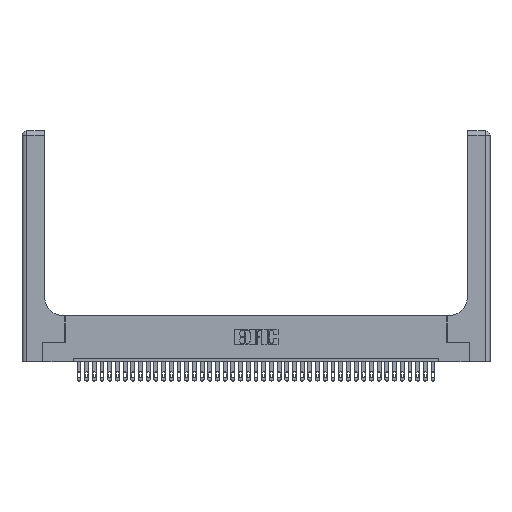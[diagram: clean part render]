
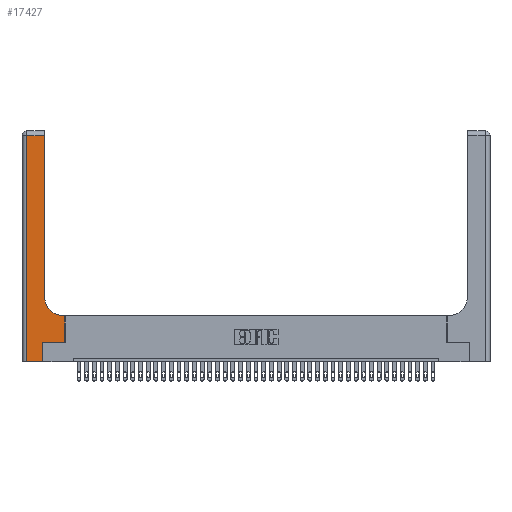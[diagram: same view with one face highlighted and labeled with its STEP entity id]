
A CAD part, top view. The second image highlights one B-rep face of the part: STEP entity #17427.
In plain terms, the highlighted planar face has unit normal (0, 0, 1).
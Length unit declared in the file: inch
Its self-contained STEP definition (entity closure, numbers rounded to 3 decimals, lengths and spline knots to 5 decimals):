
#260 = VECTOR ( 'NONE', #39578, 39.37008 ) ;
#973 = DIRECTION ( 'NONE',  ( -1., 0., 0. ) ) ;
#1329 = CARTESIAN_POINT ( 'NONE',  ( 0., 0., 0.37 ) ) ;
#2765 = ORIENTED_EDGE ( 'NONE', *, *, #15605, .T. ) ;
#3340 = ORIENTED_EDGE ( 'NONE', *, *, #33267, .T. ) ;
#4888 = CARTESIAN_POINT ( 'NONE',  ( 0.5415, 0.6, 0.37 ) ) ;
#5018 = VERTEX_POINT ( 'NONE', #16347 ) ;
#5413 = CARTESIAN_POINT ( 'NONE',  ( 0.269, 0., 0.37 ) ) ;
#5514 = ORIENTED_EDGE ( 'NONE', *, *, #7257, .T. ) ;
#5590 = CARTESIAN_POINT ( 'NONE',  ( 0., 3., 0.37 ) ) ;
#6979 = CARTESIAN_POINT ( 'NONE',  ( 0.06, 0., 0.37 ) ) ;
#7206 = EDGE_CURVE ( 'NONE', #26803, #15564, #38895, .T. ) ;
#7257 = EDGE_CURVE ( 'NONE', #11593, #26803, #11044, .T. ) ;
#7399 = VECTOR ( 'NONE', #9250, 39.37008 ) ;
#7407 = DIRECTION ( 'NONE',  ( 1., 0., 0. ) ) ;
#7465 = CARTESIAN_POINT ( 'NONE',  ( 0.269, 0.25, 0.37 ) ) ;
#8481 = DIRECTION ( 'NONE',  ( 1., 0., 0. ) ) ;
#8624 = AXIS2_PLACEMENT_3D ( 'NONE', #5590, #21650, #32143 ) ;
#9064 = DIRECTION ( 'NONE',  ( 0., -1., 0. ) ) ;
#9250 = DIRECTION ( 'NONE',  ( 0., 1., 0. ) ) ;
#9526 = EDGE_CURVE ( 'NONE', #18075, #10929, #9909, .T. ) ;
#9619 = CARTESIAN_POINT ( 'NONE',  ( 0.269, 0.25, 0.37 ) ) ;
#9711 = AXIS2_PLACEMENT_3D ( 'NONE', #26920, #11451, #8481 ) ;
#9909 = LINE ( 'NONE', #14448, #29654 ) ;
#9995 = CARTESIAN_POINT ( 'NONE',  ( 0.06, 2.94, 0.37 ) ) ;
#10929 = VERTEX_POINT ( 'NONE', #25604 ) ;
#11044 = LINE ( 'NONE', #21065, #27843 ) ;
#11447 = FACE_OUTER_BOUND ( 'NONE', #23455, .T. ) ;
#11451 = DIRECTION ( 'NONE',  ( 0., 0., -1. ) ) ;
#11593 = VERTEX_POINT ( 'NONE', #9995 ) ;
#11701 = ORIENTED_EDGE ( 'NONE', *, *, #29765, .T. ) ;
#13202 = ORIENTED_EDGE ( 'NONE', *, *, #7206, .T. ) ;
#13332 = VERTEX_POINT ( 'NONE', #7465 ) ;
#13563 = ORIENTED_EDGE ( 'NONE', *, *, #9526, .T. ) ;
#14448 = CARTESIAN_POINT ( 'NONE',  ( 0.2915, 3., 0.37 ) ) ;
#14569 = EDGE_CURVE ( 'NONE', #16712, #23626, #25360, .T. ) ;
#14992 = CARTESIAN_POINT ( 'NONE',  ( 0.269, 0., 0.37 ) ) ;
#15546 = ORIENTED_EDGE ( 'NONE', *, *, #37842, .T. ) ;
#15564 = VERTEX_POINT ( 'NONE', #14992 ) ;
#15605 = EDGE_CURVE ( 'NONE', #15564, #13332, #25283, .T. ) ;
#16292 = ORIENTED_EDGE ( 'NONE', *, *, #14569, .T. ) ;
#16347 = CARTESIAN_POINT ( 'NONE',  ( 0.5585, 0.25, 0.37 ) ) ;
#16712 = VERTEX_POINT ( 'NONE', #19251 ) ;
#16969 = ORIENTED_EDGE ( 'NONE', *, *, #19498, .T. ) ;
#17427 = ADVANCED_FACE ( 'NONE', ( #11447 ), #22324, .F. ) ;
#17683 = LINE ( 'NONE', #39328, #260 ) ;
#18075 = VERTEX_POINT ( 'NONE', #34921 ) ;
#19251 = CARTESIAN_POINT ( 'NONE',  ( 0.5585, 0.6, 0.37 ) ) ;
#19498 = EDGE_CURVE ( 'NONE', #5018, #16712, #25696, .T. ) ;
#21065 = CARTESIAN_POINT ( 'NONE',  ( 0.06, 3., 0.37 ) ) ;
#21650 = DIRECTION ( 'NONE',  ( 0., 0., -1. ) ) ;
#22156 = CIRCLE ( 'NONE', #9711, 0.25 ) ;
#22324 = PLANE ( 'NONE',  #8624 ) ;
#23455 = EDGE_LOOP ( 'NONE', ( #13563, #11701, #5514, #13202, #2765, #15546, #16969, #16292, #3340 ) ) ;
#23626 = VERTEX_POINT ( 'NONE', #4888 ) ;
#25283 = LINE ( 'NONE', #5413, #37274 ) ;
#25360 = LINE ( 'NONE', #27559, #35457 ) ;
#25442 = VECTOR ( 'NONE', #7407, 39.37008 ) ;
#25604 = CARTESIAN_POINT ( 'NONE',  ( 0.2915, 2.94, 0.37 ) ) ;
#25696 = LINE ( 'NONE', #35453, #7399 ) ;
#26803 = VERTEX_POINT ( 'NONE', #6979 ) ;
#26920 = CARTESIAN_POINT ( 'NONE',  ( 0.5415, 0.85, 0.37 ) ) ;
#27559 = CARTESIAN_POINT ( 'NONE',  ( 0.2915, 0.6, 0.37 ) ) ;
#27843 = VECTOR ( 'NONE', #9064, 39.37008 ) ;
#28445 = VECTOR ( 'NONE', #31257, 39.37008 ) ;
#29654 = VECTOR ( 'NONE', #32841, 39.37008 ) ;
#29765 = EDGE_CURVE ( 'NONE', #10929, #11593, #17683, .T. ) ;
#31257 = DIRECTION ( 'NONE',  ( 1., 0., 0. ) ) ;
#32143 = DIRECTION ( 'NONE',  ( -1., 0., 0. ) ) ;
#32841 = DIRECTION ( 'NONE',  ( 0., 1., 0. ) ) ;
#33267 = EDGE_CURVE ( 'NONE', #23626, #18075, #22156, .T. ) ;
#34921 = CARTESIAN_POINT ( 'NONE',  ( 0.2915, 0.85, 0.37 ) ) ;
#35453 = CARTESIAN_POINT ( 'NONE',  ( 0.5585, 0.25, 0.37 ) ) ;
#35457 = VECTOR ( 'NONE', #973, 39.37008 ) ;
#36042 = DIRECTION ( 'NONE',  ( 0., 1., 0. ) ) ;
#37274 = VECTOR ( 'NONE', #36042, 39.37008 ) ;
#37842 = EDGE_CURVE ( 'NONE', #13332, #5018, #38060, .T. ) ;
#38060 = LINE ( 'NONE', #9619, #28445 ) ;
#38895 = LINE ( 'NONE', #1329, #25442 ) ;
#39328 = CARTESIAN_POINT ( 'NONE',  ( 0., 2.94, 0.37 ) ) ;
#39578 = DIRECTION ( 'NONE',  ( -1., 0., 0. ) ) ;
